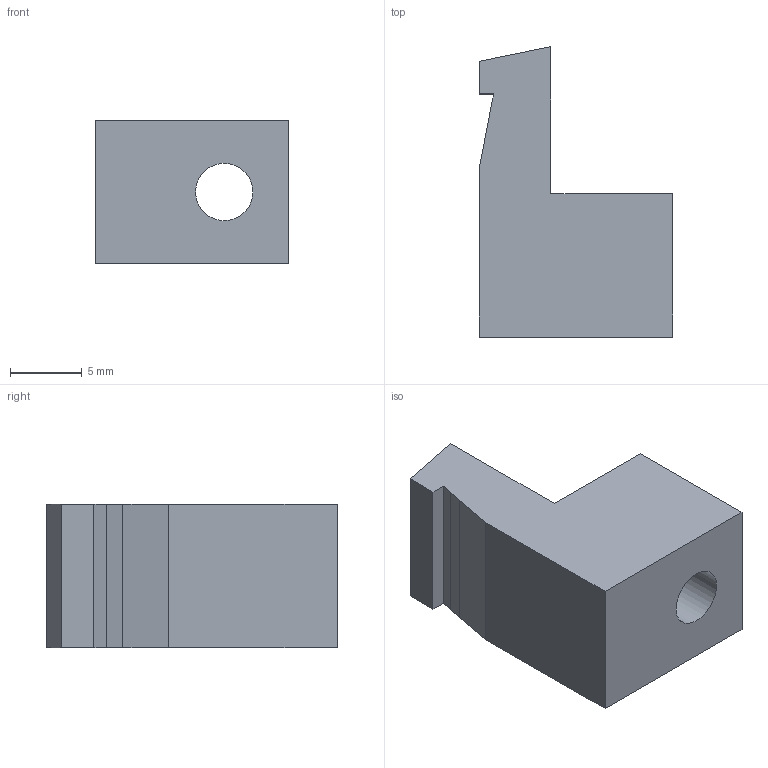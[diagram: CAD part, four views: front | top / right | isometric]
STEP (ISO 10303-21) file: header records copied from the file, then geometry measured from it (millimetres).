
FILE_DESCRIPTION (( 'STEP AP203' ), '1' );
FILE_NAME ('WTF-9_feed_ramp.STEP', '2020-05-09T10:15:00', ( '' ), ( '' ), 'SwSTEP 2.0', 'SolidWorks 2016', '' );
FILE_SCHEMA (( 'CONFIG_CONTROL_DESIGN' ));
Length unit declared in the file: millimetre
Products named in the file (2): WTF-9_feed_ramp; WTF9 V1 FINAL
Assembly tree (1 placements, depth 2):
  WTF-9_feed_ramp
    WTF9 V1 FINAL
Bounding box: 13.5 x 20.24 x 10 mm (x, y, z)
Volume: 1684.5 mm3; surface area: 1139.3 mm2
Topology: 1 solids, 1 shells, 15 faces, 39 edges, 26 vertices
Faces by surface type: plane 14, cylinder 1
Full cylindrical faces by diameter (mm): 4 x1
Entity records: 650 total; most frequent: CARTESIAN_POINT 83, DIRECTION 78, ORIENTED_EDGE 76, EDGE_CURVE 38, VECTOR 36, LINE 36, VERTEX_POINT 26, AXIS2_PLACEMENT_3D 21
